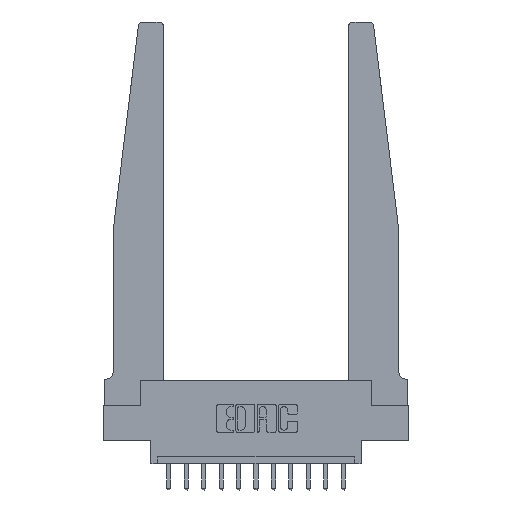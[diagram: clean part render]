
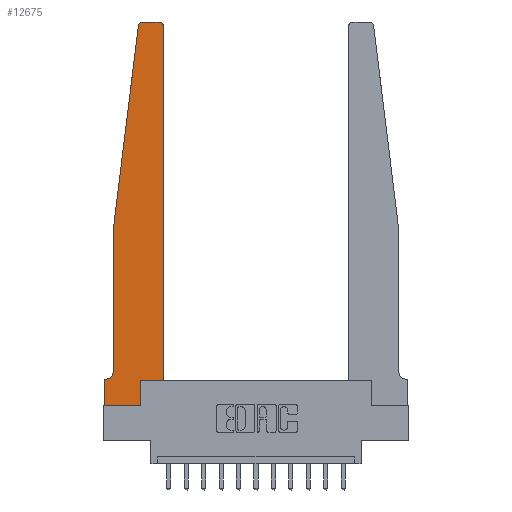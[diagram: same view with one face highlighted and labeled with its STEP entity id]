
A CAD part, top view. The second image highlights one B-rep face of the part: STEP entity #12675.
In plain terms, the highlighted planar face has unit normal (0, 0, 1).
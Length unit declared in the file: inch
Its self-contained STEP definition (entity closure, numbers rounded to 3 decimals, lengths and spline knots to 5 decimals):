
#139 = ORIENTED_EDGE ( 'NONE', *, *, #1186, .T. ) ;
#326 = ORIENTED_EDGE ( 'NONE', *, *, #6510, .T. ) ;
#590 = CARTESIAN_POINT ( 'NONE',  ( 0.065, 0.2375, 0.37 ) ) ;
#704 = PLANE ( 'NONE',  #7213 ) ;
#714 = EDGE_CURVE ( 'NONE', #13341, #6446, #5089, .T. ) ;
#936 = CARTESIAN_POINT ( 'NONE',  ( 0.2605, 0.18, 0.37 ) ) ;
#1141 = AXIS2_PLACEMENT_3D ( 'NONE', #9732, #4828, #3407 ) ;
#1186 = EDGE_CURVE ( 'NONE', #1816, #9206, #8967, .T. ) ;
#1187 = DIRECTION ( 'NONE',  ( 1., 0., 0. ) ) ;
#1400 = LINE ( 'NONE', #7944, #11161 ) ;
#1816 = VERTEX_POINT ( 'NONE', #12224 ) ;
#1852 = VECTOR ( 'NONE', #12221, 39.37008 ) ;
#1909 = DIRECTION ( 'NONE',  ( 1., 0., 0. ) ) ;
#2076 = DIRECTION ( 'NONE',  ( 0., 0., 1. ) ) ;
#2207 = AXIS2_PLACEMENT_3D ( 'NONE', #5911, #2076, #1909 ) ;
#2626 = EDGE_CURVE ( 'NONE', #13977, #12678, #3426, .T. ) ;
#2862 = LINE ( 'NONE', #4194, #5042 ) ;
#3165 = CARTESIAN_POINT ( 'NONE',  ( 0.065, 0.1875, 0.37 ) ) ;
#3177 = CARTESIAN_POINT ( 'NONE',  ( 0., 0., 0.37 ) ) ;
#3246 = VECTOR ( 'NONE', #4511, 39.37008 ) ;
#3407 = DIRECTION ( 'NONE',  ( -1., 0., 0. ) ) ;
#3426 = LINE ( 'NONE', #8496, #11959 ) ;
#3683 = CARTESIAN_POINT ( 'NONE',  ( 0.065, 1.25, 0.37 ) ) ;
#3736 = DIRECTION ( 'NONE',  ( 1., 0., 0. ) ) ;
#3855 = DIRECTION ( 'NONE',  ( 0., 0., 1. ) ) ;
#4194 = CARTESIAN_POINT ( 'NONE',  ( 0.425, 0.18, 0.37 ) ) ;
#4483 = EDGE_CURVE ( 'NONE', #12678, #16081, #11272, .T. ) ;
#4511 = DIRECTION ( 'NONE',  ( -1., 0., 0. ) ) ;
#4594 = CARTESIAN_POINT ( 'NONE',  ( 0.24675, 2.72367, 0.37 ) ) ;
#4828 = DIRECTION ( 'NONE',  ( 0., 0., -1. ) ) ;
#5042 = VECTOR ( 'NONE', #10844, 39.37008 ) ;
#5089 = CIRCLE ( 'NONE', #14670, 0.03 ) ;
#5823 = CARTESIAN_POINT ( 'NONE',  ( 0.425, 2.72, 0.37 ) ) ;
#5911 = CARTESIAN_POINT ( 'NONE',  ( 0.395, 2.72, 0.37 ) ) ;
#6446 = VERTEX_POINT ( 'NONE', #4594 ) ;
#6466 = ORIENTED_EDGE ( 'NONE', *, *, #9750, .T. ) ;
#6474 = CARTESIAN_POINT ( 'NONE',  ( 0.065, 1.25, 0.37 ) ) ;
#6494 = CARTESIAN_POINT ( 'NONE',  ( 0.27653, 2.75, 0.37 ) ) ;
#6510 = EDGE_CURVE ( 'NONE', #12570, #11698, #9644, .T. ) ;
#6692 = CARTESIAN_POINT ( 'NONE',  ( 0.015, 0.1875, 0.37 ) ) ;
#6849 = VECTOR ( 'NONE', #9924, 39.37008 ) ;
#6903 = VERTEX_POINT ( 'NONE', #590 ) ;
#6948 = VECTOR ( 'NONE', #15845, 39.37008 ) ;
#7092 = ORIENTED_EDGE ( 'NONE', *, *, #4483, .T. ) ;
#7213 = AXIS2_PLACEMENT_3D ( 'NONE', #13367, #8006, #9494 ) ;
#7744 = ORIENTED_EDGE ( 'NONE', *, *, #714, .T. ) ;
#7944 = CARTESIAN_POINT ( 'NONE',  ( 0.25, 2.75, 0.37 ) ) ;
#8006 = DIRECTION ( 'NONE',  ( 0., 0., 1. ) ) ;
#8308 = CIRCLE ( 'NONE', #1141, 0.05 ) ;
#8446 = ORIENTED_EDGE ( 'NONE', *, *, #10086, .T. ) ;
#8496 = CARTESIAN_POINT ( 'NONE',  ( 0., 0., 0.37 ) ) ;
#8967 = LINE ( 'NONE', #15154, #11446 ) ;
#9130 = VECTOR ( 'NONE', #15052, 39.37008 ) ;
#9206 = VERTEX_POINT ( 'NONE', #5823 ) ;
#9482 = EDGE_CURVE ( 'NONE', #13625, #13341, #1400, .T. ) ;
#9494 = DIRECTION ( 'NONE',  ( 1., 0., 0. ) ) ;
#9644 = LINE ( 'NONE', #3165, #3246 ) ;
#9732 = CARTESIAN_POINT ( 'NONE',  ( 0.015, 0.2375, 0.37 ) ) ;
#9749 = CARTESIAN_POINT ( 'NONE',  ( 0., 0., 0.37 ) ) ;
#9750 = EDGE_CURVE ( 'NONE', #6446, #10506, #16352, .T. ) ;
#9924 = DIRECTION ( 'NONE',  ( 0., 1., 0. ) ) ;
#9987 = CARTESIAN_POINT ( 'NONE',  ( 0.27653, 2.72, 0.37 ) ) ;
#10086 = EDGE_CURVE ( 'NONE', #16081, #1816, #2862, .T. ) ;
#10492 = ORIENTED_EDGE ( 'NONE', *, *, #16385, .T. ) ;
#10506 = VERTEX_POINT ( 'NONE', #13422 ) ;
#10844 = DIRECTION ( 'NONE',  ( 1., 0., 0. ) ) ;
#10967 = CARTESIAN_POINT ( 'NONE',  ( 0.395, 2.75, 0.37 ) ) ;
#11161 = VECTOR ( 'NONE', #15470, 39.37008 ) ;
#11191 = EDGE_LOOP ( 'NONE', ( #12325, #7744, #6466, #16034, #14393, #326, #11728, #12862, #7092, #8446, #139, #10492 ) ) ;
#11272 = LINE ( 'NONE', #14052, #6849 ) ;
#11446 = VECTOR ( 'NONE', #15325, 39.37008 ) ;
#11698 = VERTEX_POINT ( 'NONE', #13357 ) ;
#11728 = ORIENTED_EDGE ( 'NONE', *, *, #12691, .T. ) ;
#11959 = VECTOR ( 'NONE', #3736, 39.37008 ) ;
#12221 = DIRECTION ( 'NONE',  ( -0.122, -0.992, 0. ) ) ;
#12224 = CARTESIAN_POINT ( 'NONE',  ( 0.425, 0.18, 0.37 ) ) ;
#12325 = ORIENTED_EDGE ( 'NONE', *, *, #9482, .T. ) ;
#12487 = LINE ( 'NONE', #6474, #9130 ) ;
#12570 = VERTEX_POINT ( 'NONE', #6692 ) ;
#12675 = ADVANCED_FACE ( 'NONE', ( #15765 ), #704, .T. ) ;
#12678 = VERTEX_POINT ( 'NONE', #14457 ) ;
#12691 = EDGE_CURVE ( 'NONE', #11698, #13977, #13129, .T. ) ;
#12862 = ORIENTED_EDGE ( 'NONE', *, *, #2626, .T. ) ;
#13129 = LINE ( 'NONE', #3177, #6948 ) ;
#13341 = VERTEX_POINT ( 'NONE', #6494 ) ;
#13357 = CARTESIAN_POINT ( 'NONE',  ( 0., 0.1875, 0.37 ) ) ;
#13367 = CARTESIAN_POINT ( 'NONE',  ( 0., 0.1875, 0.37 ) ) ;
#13422 = CARTESIAN_POINT ( 'NONE',  ( 0.065, 1.25, 0.37 ) ) ;
#13625 = VERTEX_POINT ( 'NONE', #10967 ) ;
#13977 = VERTEX_POINT ( 'NONE', #9749 ) ;
#14052 = CARTESIAN_POINT ( 'NONE',  ( 0.2605, 0.18, 0.37 ) ) ;
#14393 = ORIENTED_EDGE ( 'NONE', *, *, #14455, .T. ) ;
#14455 = EDGE_CURVE ( 'NONE', #6903, #12570, #8308, .T. ) ;
#14457 = CARTESIAN_POINT ( 'NONE',  ( 0.2605, 0., 0.37 ) ) ;
#14670 = AXIS2_PLACEMENT_3D ( 'NONE', #9987, #3855, #1187 ) ;
#14727 = CIRCLE ( 'NONE', #2207, 0.03 ) ;
#15052 = DIRECTION ( 'NONE',  ( 0., -1., 0. ) ) ;
#15092 = EDGE_CURVE ( 'NONE', #10506, #6903, #12487, .T. ) ;
#15154 = CARTESIAN_POINT ( 'NONE',  ( 0.425, 0.18, 0.37 ) ) ;
#15325 = DIRECTION ( 'NONE',  ( 0., 1., 0. ) ) ;
#15470 = DIRECTION ( 'NONE',  ( -1., 0., 0. ) ) ;
#15765 = FACE_OUTER_BOUND ( 'NONE', #11191, .T. ) ;
#15845 = DIRECTION ( 'NONE',  ( 0., -1., 0. ) ) ;
#16034 = ORIENTED_EDGE ( 'NONE', *, *, #15092, .T. ) ;
#16081 = VERTEX_POINT ( 'NONE', #936 ) ;
#16352 = LINE ( 'NONE', #3683, #1852 ) ;
#16385 = EDGE_CURVE ( 'NONE', #9206, #13625, #14727, .T. ) ;
